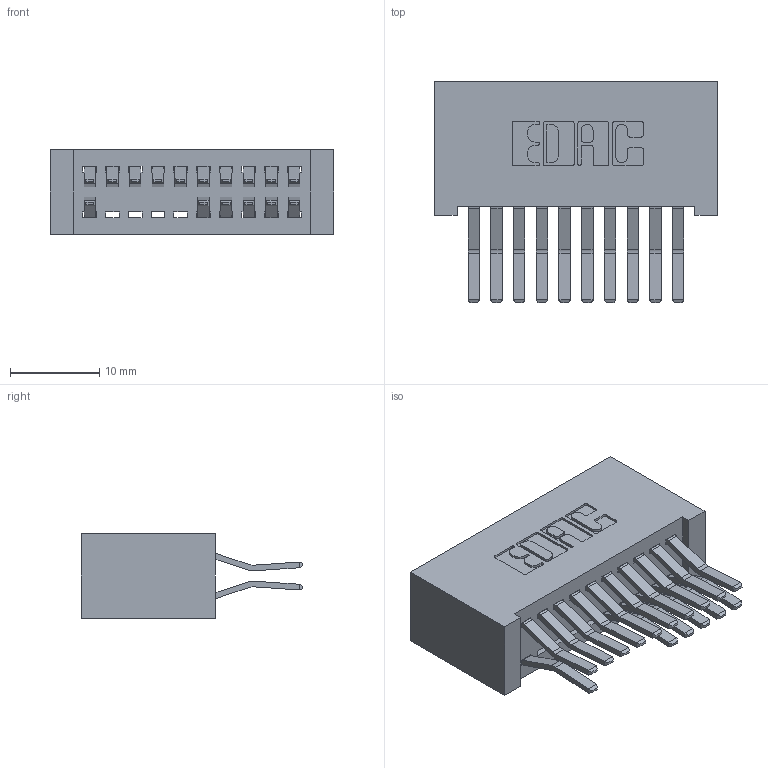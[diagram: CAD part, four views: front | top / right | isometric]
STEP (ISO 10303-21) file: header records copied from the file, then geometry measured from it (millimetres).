
FILE_DESCRIPTION (( 'STEP AP203' ), '1' );
FILE_NAME ('392-020-560-201.STEP', '2018-08-15T07:27:40', ( '' ), ( '' ), 'SwSTEP 2.0', 'SolidWorks 2016', '' );
FILE_SCHEMA (( 'CONFIG_CONTROL_DESIGN' ));
Length unit declared in the file: inch
Products named in the file (3): 342 Part_Lugless; 345-292-001_560 Tail; 392-020-560-201
Assembly tree (17 placements, depth 2):
  392-020-560-201
    342 Part_Lugless
    345-292-001_560 Tail  x16
Bounding box: 31.65 x 24.78 x 9.4 mm (x, y, z)
Volume: 3200.7 mm3; surface area: 4920.6 mm2
Topology: 17 solids, 17 shells, 990 faces, 2935 edges, 1934 vertices
Faces by surface type: plane 662, cylinder 328
Entity records: 10123 total; most frequent: CARTESIAN_POINT 1730, ORIENTED_EDGE 1670, DIRECTION 1527, EDGE_CURVE 835, LINE 711, VECTOR 711, VERTEX_POINT 554, AXIS2_PLACEMENT_3D 408
